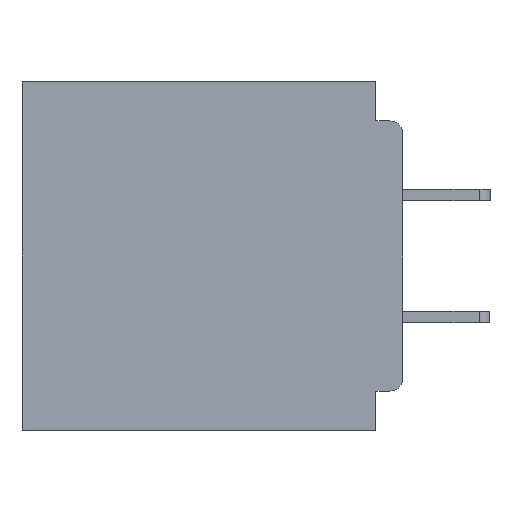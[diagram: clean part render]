
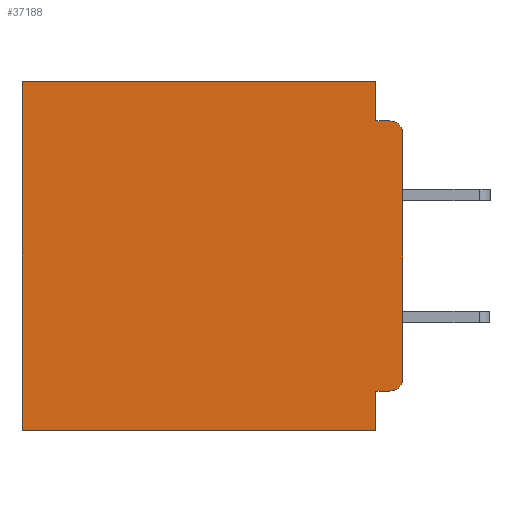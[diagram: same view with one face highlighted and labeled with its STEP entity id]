
A CAD part, left-side view. The second image highlights one B-rep face of the part: STEP entity #37188.
In plain terms, the highlighted planar face has unit normal (-1, 0, 0).
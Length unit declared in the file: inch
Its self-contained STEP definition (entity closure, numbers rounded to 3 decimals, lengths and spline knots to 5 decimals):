
#361 = VERTEX_POINT ( 'NONE', #2311 ) ;
#1118 = LINE ( 'NONE', #55294, #36225 ) ;
#1137 = LINE ( 'NONE', #9274, #56889 ) ;
#2311 = CARTESIAN_POINT ( 'NONE',  ( 0.3, 0.015, -0.045 ) ) ;
#2999 = CARTESIAN_POINT ( 'NONE',  ( 0.3, 0.437, 0. ) ) ;
#3495 = AXIS2_PLACEMENT_3D ( 'NONE', #24186, #55023, #28652 ) ;
#8865 = CIRCLE ( 'NONE', #3495, 0.015 ) ;
#9274 = CARTESIAN_POINT ( 'NONE',  ( 0.3, 0.031, -0.4 ) ) ;
#9807 = EDGE_CURVE ( 'NONE', #42140, #47520, #43880, .T. ) ;
#12023 = DIRECTION ( 'NONE',  ( 0., 0., -1. ) ) ;
#13660 = DIRECTION ( 'NONE',  ( 0., 0., -1. ) ) ;
#14176 = ORIENTED_EDGE ( 'NONE', *, *, #9807, .F. ) ;
#14613 = LINE ( 'NONE', #19402, #48409 ) ;
#15423 = EDGE_CURVE ( 'NONE', #36816, #27259, #55273, .T. ) ;
#15568 = CARTESIAN_POINT ( 'NONE',  ( 0.3, 0., -0.4 ) ) ;
#15967 = ORIENTED_EDGE ( 'NONE', *, *, #50381, .T. ) ;
#16049 = VERTEX_POINT ( 'NONE', #31727 ) ;
#16824 = CARTESIAN_POINT ( 'NONE',  ( 0.3, 0.437, -0.4 ) ) ;
#18274 = EDGE_CURVE ( 'NONE', #42140, #361, #38504, .T. ) ;
#18292 = DIRECTION ( 'NONE',  ( 0., -1., 0. ) ) ;
#19402 = CARTESIAN_POINT ( 'NONE',  ( 0.3, 0.437, -0.4 ) ) ;
#19437 = FACE_OUTER_BOUND ( 'NONE', #48060, .T. ) ;
#20802 = ORIENTED_EDGE ( 'NONE', *, *, #18274, .T. ) ;
#21491 = AXIS2_PLACEMENT_3D ( 'NONE', #42653, #38402, #12023 ) ;
#21702 = VERTEX_POINT ( 'NONE', #2999 ) ;
#22737 = EDGE_CURVE ( 'NONE', #41104, #16049, #1118, .T. ) ;
#23819 = DIRECTION ( 'NONE',  ( 0., 0., -1. ) ) ;
#24186 = CARTESIAN_POINT ( 'NONE',  ( 0.3, 0.015, -0.34 ) ) ;
#24410 = DIRECTION ( 'NONE',  ( -1., 0., 0. ) ) ;
#25330 = DIRECTION ( 'NONE',  ( 0., 0., -1. ) ) ;
#25515 = ORIENTED_EDGE ( 'NONE', *, *, #28462, .T. ) ;
#27259 = VERTEX_POINT ( 'NONE', #16824 ) ;
#27273 = CARTESIAN_POINT ( 'NONE',  ( 0.3, 0.015, -0.355 ) ) ;
#27394 = CARTESIAN_POINT ( 'NONE',  ( 0.3, 0., -0.34 ) ) ;
#27669 = CARTESIAN_POINT ( 'NONE',  ( 0.3, 0.031, 0. ) ) ;
#28462 = EDGE_CURVE ( 'NONE', #41104, #47520, #8865, .T. ) ;
#28652 = DIRECTION ( 'NONE',  ( 0., 0., -1. ) ) ;
#28936 = DIRECTION ( 'NONE',  ( 0., 1., 0. ) ) ;
#30416 = EDGE_CURVE ( 'NONE', #53825, #38671, #44458, .T. ) ;
#30552 = ORIENTED_EDGE ( 'NONE', *, *, #22737, .F. ) ;
#31727 = CARTESIAN_POINT ( 'NONE',  ( 0.3, 0.031, -0.355 ) ) ;
#31896 = VECTOR ( 'NONE', #39635, 39.37008 ) ;
#34295 = ORIENTED_EDGE ( 'NONE', *, *, #30416, .F. ) ;
#35407 = CARTESIAN_POINT ( 'NONE',  ( 0.3, 0., -0.4 ) ) ;
#35852 = CARTESIAN_POINT ( 'NONE',  ( 0.3, 0., -0.045 ) ) ;
#36225 = VECTOR ( 'NONE', #28936, 39.37008 ) ;
#36816 = VERTEX_POINT ( 'NONE', #48067 ) ;
#37188 = ADVANCED_FACE ( 'NONE', ( #19437 ), #55916, .F. ) ;
#37343 = DIRECTION ( 'NONE',  ( 0., 1., 0. ) ) ;
#37527 = CARTESIAN_POINT ( 'NONE',  ( 0.3, 0., 0. ) ) ;
#38402 = DIRECTION ( 'NONE',  ( 1., 0., 0. ) ) ;
#38504 = CIRCLE ( 'NONE', #42174, 0.015 ) ;
#38671 = VERTEX_POINT ( 'NONE', #39592 ) ;
#39407 = EDGE_CURVE ( 'NONE', #38671, #361, #48626, .T. ) ;
#39592 = CARTESIAN_POINT ( 'NONE',  ( 0.3, 0.031, -0.045 ) ) ;
#39635 = DIRECTION ( 'NONE',  ( 0., 1., 0. ) ) ;
#40694 = ORIENTED_EDGE ( 'NONE', *, *, #44565, .F. ) ;
#41104 = VERTEX_POINT ( 'NONE', #27273 ) ;
#42140 = VERTEX_POINT ( 'NONE', #42980 ) ;
#42174 = AXIS2_PLACEMENT_3D ( 'NONE', #50831, #24410, #55235 ) ;
#42653 = CARTESIAN_POINT ( 'NONE',  ( 0.3, 0., -0.4 ) ) ;
#42980 = CARTESIAN_POINT ( 'NONE',  ( 0.3, 0., -0.06 ) ) ;
#43880 = LINE ( 'NONE', #15568, #52813 ) ;
#44458 = LINE ( 'NONE', #47340, #54759 ) ;
#44565 = EDGE_CURVE ( 'NONE', #16049, #36816, #1137, .T. ) ;
#44840 = EDGE_CURVE ( 'NONE', #53825, #21702, #56550, .T. ) ;
#44869 = VECTOR ( 'NONE', #37343, 39.37008 ) ;
#47237 = VECTOR ( 'NONE', #18292, 39.37008 ) ;
#47340 = CARTESIAN_POINT ( 'NONE',  ( 0.3, 0.031, 0. ) ) ;
#47520 = VERTEX_POINT ( 'NONE', #27394 ) ;
#48060 = EDGE_LOOP ( 'NONE', ( #14176, #20802, #53901, #34295, #50506, #15967, #49207, #40694, #30552, #25515 ) ) ;
#48067 = CARTESIAN_POINT ( 'NONE',  ( 0.3, 0.031, -0.4 ) ) ;
#48409 = VECTOR ( 'NONE', #23819, 39.37008 ) ;
#48626 = LINE ( 'NONE', #35852, #47237 ) ;
#49207 = ORIENTED_EDGE ( 'NONE', *, *, #15423, .F. ) ;
#50381 = EDGE_CURVE ( 'NONE', #21702, #27259, #14613, .T. ) ;
#50506 = ORIENTED_EDGE ( 'NONE', *, *, #44840, .T. ) ;
#50831 = CARTESIAN_POINT ( 'NONE',  ( 0.3, 0.015, -0.06 ) ) ;
#52813 = VECTOR ( 'NONE', #55251, 39.37008 ) ;
#53825 = VERTEX_POINT ( 'NONE', #27669 ) ;
#53901 = ORIENTED_EDGE ( 'NONE', *, *, #39407, .F. ) ;
#54759 = VECTOR ( 'NONE', #25330, 39.37008 ) ;
#55023 = DIRECTION ( 'NONE',  ( -1., 0., 0. ) ) ;
#55235 = DIRECTION ( 'NONE',  ( 0., 0., -1. ) ) ;
#55251 = DIRECTION ( 'NONE',  ( 0., 0., -1. ) ) ;
#55273 = LINE ( 'NONE', #35407, #31896 ) ;
#55294 = CARTESIAN_POINT ( 'NONE',  ( 0.3, 0., -0.355 ) ) ;
#55916 = PLANE ( 'NONE',  #21491 ) ;
#56550 = LINE ( 'NONE', #37527, #44869 ) ;
#56889 = VECTOR ( 'NONE', #13660, 39.37008 ) ;
